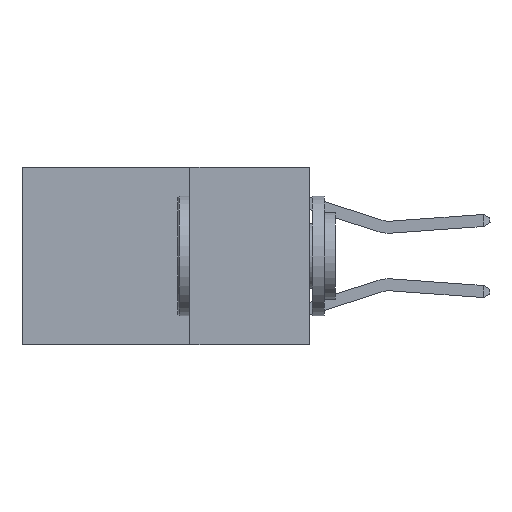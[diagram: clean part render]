
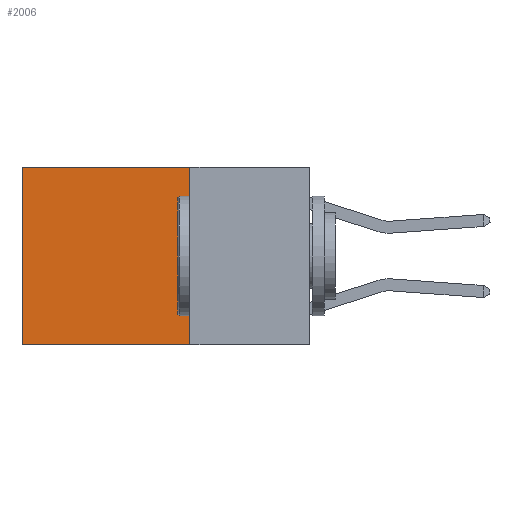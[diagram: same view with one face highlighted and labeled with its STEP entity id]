
A CAD part, left-side view. The second image highlights one B-rep face of the part: STEP entity #2006.
In plain terms, the highlighted planar face has unit normal (-1, 0, 0).
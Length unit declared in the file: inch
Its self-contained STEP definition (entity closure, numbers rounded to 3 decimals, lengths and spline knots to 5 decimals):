
#20 = CARTESIAN_POINT ( 'NONE',  ( 0.2625, 0.6, 0. ) ) ;
#427 = EDGE_CURVE ( 'NONE', #2692, #556, #6445, .T. ) ;
#556 = VERTEX_POINT ( 'NONE', #2554 ) ;
#825 = CARTESIAN_POINT ( 'NONE',  ( 0.2625, 0.25, 0. ) ) ;
#1094 = AXIS2_PLACEMENT_3D ( 'NONE', #7330, #4288, #9528 ) ;
#1127 = VERTEX_POINT ( 'NONE', #20 ) ;
#2006 = ADVANCED_FACE ( 'NONE', ( #8799 ), #8089, .F. ) ;
#2397 = ORIENTED_EDGE ( 'NONE', *, *, #5104, .T. ) ;
#2492 = ORIENTED_EDGE ( 'NONE', *, *, #7271, .F. ) ;
#2554 = CARTESIAN_POINT ( 'NONE',  ( 0.2625, 0.6, -0.37 ) ) ;
#2692 = VERTEX_POINT ( 'NONE', #5341 ) ;
#2903 = VECTOR ( 'NONE', #9478, 39.37008 ) ;
#4288 = DIRECTION ( 'NONE',  ( 1., 0., 0. ) ) ;
#4381 = EDGE_LOOP ( 'NONE', ( #4767, #5373, #2492, #2397 ) ) ;
#4767 = ORIENTED_EDGE ( 'NONE', *, *, #9286, .T. ) ;
#5101 = LINE ( 'NONE', #8725, #2903 ) ;
#5104 = EDGE_CURVE ( 'NONE', #9003, #1127, #8663, .T. ) ;
#5150 = DIRECTION ( 'NONE',  ( 0., 1., 0. ) ) ;
#5341 = CARTESIAN_POINT ( 'NONE',  ( 0.2625, 0.25, -0.37 ) ) ;
#5373 = ORIENTED_EDGE ( 'NONE', *, *, #427, .F. ) ;
#5728 = DIRECTION ( 'NONE',  ( 0., 0., -1. ) ) ;
#6202 = VECTOR ( 'NONE', #7592, 39.37008 ) ;
#6445 = LINE ( 'NONE', #7624, #6202 ) ;
#6491 = CARTESIAN_POINT ( 'NONE',  ( 0.2625, 0.25, 0. ) ) ;
#6500 = VECTOR ( 'NONE', #5150, 39.37008 ) ;
#7271 = EDGE_CURVE ( 'NONE', #9003, #2692, #9287, .T. ) ;
#7330 = CARTESIAN_POINT ( 'NONE',  ( 0.2625, 0.25, 0. ) ) ;
#7387 = VECTOR ( 'NONE', #5728, 39.37008 ) ;
#7592 = DIRECTION ( 'NONE',  ( 0., 1., 0. ) ) ;
#7624 = CARTESIAN_POINT ( 'NONE',  ( 0.2625, 0.25, -0.37 ) ) ;
#8089 = PLANE ( 'NONE',  #1094 ) ;
#8663 = LINE ( 'NONE', #9572, #6500 ) ;
#8725 = CARTESIAN_POINT ( 'NONE',  ( 0.2625, 0.6, 0. ) ) ;
#8799 = FACE_OUTER_BOUND ( 'NONE', #4381, .T. ) ;
#9003 = VERTEX_POINT ( 'NONE', #825 ) ;
#9286 = EDGE_CURVE ( 'NONE', #1127, #556, #5101, .T. ) ;
#9287 = LINE ( 'NONE', #6491, #7387 ) ;
#9478 = DIRECTION ( 'NONE',  ( 0., 0., -1. ) ) ;
#9528 = DIRECTION ( 'NONE',  ( 0., 0., -1. ) ) ;
#9572 = CARTESIAN_POINT ( 'NONE',  ( 0.2625, 0.25, 0. ) ) ;
